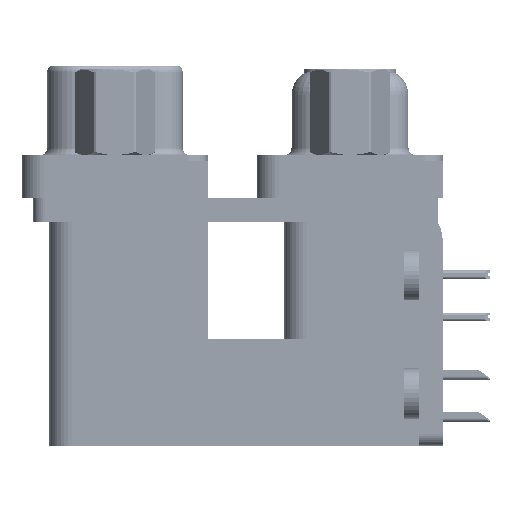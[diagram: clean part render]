
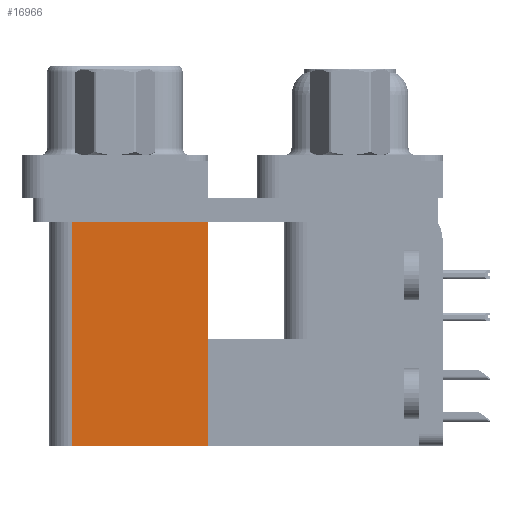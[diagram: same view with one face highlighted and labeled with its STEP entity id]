
A CAD part, left-side view. The second image highlights one B-rep face of the part: STEP entity #16966.
In plain terms, the highlighted planar face has unit normal (-1, 0, 0).
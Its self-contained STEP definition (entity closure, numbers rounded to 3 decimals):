
#198 = PLANE ( 'NONE',  #33323 ) ;
#4070 = DIRECTION ( 'NONE',  ( 0., 0., 1. ) ) ;
#4583 = ORIENTED_EDGE ( 'NONE', *, *, #52318, .F. ) ;
#5013 = CARTESIAN_POINT ( 'NONE',  ( 3.7, 9.6, -19.2 ) ) ;
#5110 = EDGE_CURVE ( 'NONE', #46629, #30741, #20545, .T. ) ;
#6798 = VERTEX_POINT ( 'NONE', #37966 ) ;
#6800 = EDGE_CURVE ( 'NONE', #35069, #46629, #57188, .T. ) ;
#8319 = VECTOR ( 'NONE', #52260, 1000. ) ;
#10158 = CARTESIAN_POINT ( 'NONE',  ( 3.7, 9.6, -2.5 ) ) ;
#10526 = EDGE_CURVE ( 'NONE', #6798, #30741, #19888, .T. ) ;
#13196 = LINE ( 'NONE', #57181, #57858 ) ;
#16966 = ADVANCED_FACE ( 'NONE', ( #48911 ), #198, .F. ) ;
#19888 = LINE ( 'NONE', #39335, #8319 ) ;
#20545 = LINE ( 'NONE', #58580, #60327 ) ;
#26896 = VECTOR ( 'NONE', #4070, 1000. ) ;
#29088 = DIRECTION ( 'NONE',  ( 0., 0., -1. ) ) ;
#30741 = VERTEX_POINT ( 'NONE', #49024 ) ;
#33323 = AXIS2_PLACEMENT_3D ( 'NONE', #53015, #43885, #29088 ) ;
#34967 = DIRECTION ( 'NONE',  ( 0., 1., 0. ) ) ;
#35069 = VERTEX_POINT ( 'NONE', #58774 ) ;
#37966 = CARTESIAN_POINT ( 'NONE',  ( 3.7, 18.8, -19.2 ) ) ;
#39335 = CARTESIAN_POINT ( 'NONE',  ( 3.7, 18.8, -19.2 ) ) ;
#43885 = DIRECTION ( 'NONE',  ( 1., 0., 0. ) ) ;
#46629 = VERTEX_POINT ( 'NONE', #10158 ) ;
#48223 = EDGE_LOOP ( 'NONE', ( #51875, #55592, #4583, #59834 ) ) ;
#48911 = FACE_OUTER_BOUND ( 'NONE', #48223, .T. ) ;
#49024 = CARTESIAN_POINT ( 'NONE',  ( 3.7, 18.8, -2.5 ) ) ;
#51875 = ORIENTED_EDGE ( 'NONE', *, *, #5110, .T. ) ;
#52260 = DIRECTION ( 'NONE',  ( 0., 0., 1. ) ) ;
#52318 = EDGE_CURVE ( 'NONE', #35069, #6798, #13196, .T. ) ;
#53015 = CARTESIAN_POINT ( 'NONE',  ( 3.7, 9.6, -19.2 ) ) ;
#55592 = ORIENTED_EDGE ( 'NONE', *, *, #10526, .F. ) ;
#57181 = CARTESIAN_POINT ( 'NONE',  ( 3.7, 9.6, -19.2 ) ) ;
#57188 = LINE ( 'NONE', #5013, #26896 ) ;
#57858 = VECTOR ( 'NONE', #61577, 1000. ) ;
#58580 = CARTESIAN_POINT ( 'NONE',  ( 3.7, 9.6, -2.5 ) ) ;
#58774 = CARTESIAN_POINT ( 'NONE',  ( 3.7, 9.6, -19.2 ) ) ;
#59834 = ORIENTED_EDGE ( 'NONE', *, *, #6800, .T. ) ;
#60327 = VECTOR ( 'NONE', #34967, 1000. ) ;
#61577 = DIRECTION ( 'NONE',  ( 0., 1., 0. ) ) ;
